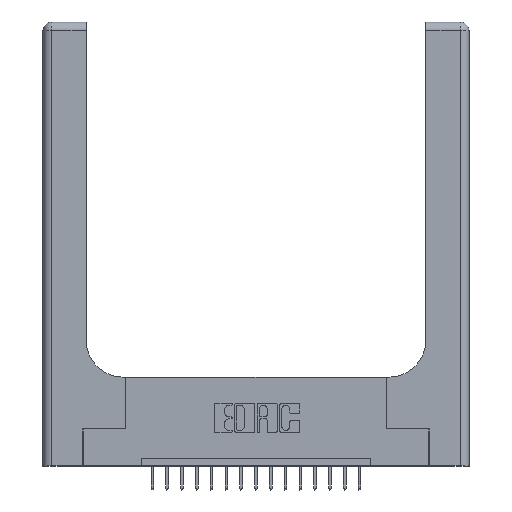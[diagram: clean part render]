
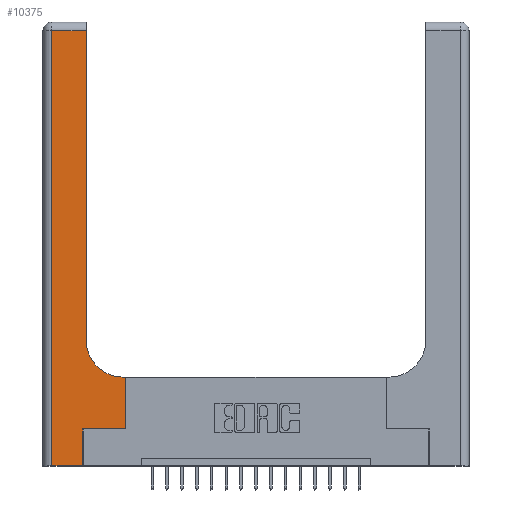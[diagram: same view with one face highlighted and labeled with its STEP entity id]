
A CAD part, top view. The second image highlights one B-rep face of the part: STEP entity #10375.
In plain terms, the highlighted planar face has unit normal (0, 0, 1).
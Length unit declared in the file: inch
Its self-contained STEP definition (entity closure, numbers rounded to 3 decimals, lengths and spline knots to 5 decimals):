
#289 = ORIENTED_EDGE ( 'NONE', *, *, #11114, .T. ) ;
#480 = DIRECTION ( 'NONE',  ( 1., 0., 0. ) ) ;
#503 = AXIS2_PLACEMENT_3D ( 'NONE', #3597, #14222, #6578 ) ;
#624 = LINE ( 'NONE', #5454, #6425 ) ;
#659 = DIRECTION ( 'NONE',  ( 1., 0., 0. ) ) ;
#871 = CARTESIAN_POINT ( 'NONE',  ( 0.269, 0., 0.37 ) ) ;
#910 = ORIENTED_EDGE ( 'NONE', *, *, #14593, .T. ) ;
#1097 = CIRCLE ( 'NONE', #3517, 0.25 ) ;
#1673 = EDGE_CURVE ( 'NONE', #16853, #19770, #10123, .T. ) ;
#1715 = DIRECTION ( 'NONE',  ( 0., 1., 0. ) ) ;
#1859 = EDGE_CURVE ( 'NONE', #10477, #11674, #624, .T. ) ;
#2254 = EDGE_CURVE ( 'NONE', #13086, #10477, #2289, .T. ) ;
#2289 = LINE ( 'NONE', #9511, #11050 ) ;
#2561 = EDGE_CURVE ( 'NONE', #14818, #2885, #15707, .T. ) ;
#2846 = ORIENTED_EDGE ( 'NONE', *, *, #12596, .T. ) ;
#2885 = VERTEX_POINT ( 'NONE', #14692 ) ;
#3455 = ORIENTED_EDGE ( 'NONE', *, *, #1859, .T. ) ;
#3517 = AXIS2_PLACEMENT_3D ( 'NONE', #14286, #15943, #480 ) ;
#3597 = CARTESIAN_POINT ( 'NONE',  ( 0., 3., 0.37 ) ) ;
#4347 = CARTESIAN_POINT ( 'NONE',  ( 0., 2.94, 0.37 ) ) ;
#4889 = LINE ( 'NONE', #10099, #17074 ) ;
#5375 = CARTESIAN_POINT ( 'NONE',  ( 0.5415, 0.6, 0.37 ) ) ;
#5384 = DIRECTION ( 'NONE',  ( 1., 0., 0. ) ) ;
#5454 = CARTESIAN_POINT ( 'NONE',  ( 0.269, 0.25, 0.37 ) ) ;
#5584 = LINE ( 'NONE', #13887, #9000 ) ;
#6143 = ORIENTED_EDGE ( 'NONE', *, *, #2561, .T. ) ;
#6267 = ORIENTED_EDGE ( 'NONE', *, *, #11590, .T. ) ;
#6387 = CARTESIAN_POINT ( 'NONE',  ( 0.06, 0., 0.37 ) ) ;
#6425 = VECTOR ( 'NONE', #5384, 39.37008 ) ;
#6578 = DIRECTION ( 'NONE',  ( -1., 0., 0. ) ) ;
#6607 = DIRECTION ( 'NONE',  ( 0., 1., 0. ) ) ;
#6799 = CARTESIAN_POINT ( 'NONE',  ( 0.5585, 0.25, 0.37 ) ) ;
#6810 = EDGE_CURVE ( 'NONE', #9966, #8165, #5584, .T. ) ;
#8165 = VERTEX_POINT ( 'NONE', #6387 ) ;
#8509 = VECTOR ( 'NONE', #6607, 39.37008 ) ;
#9000 = VECTOR ( 'NONE', #18345, 39.37008 ) ;
#9511 = CARTESIAN_POINT ( 'NONE',  ( 0.269, 0., 0.37 ) ) ;
#9547 = DIRECTION ( 'NONE',  ( -1., 0., 0. ) ) ;
#9689 = CARTESIAN_POINT ( 'NONE',  ( 0.2915, 0.6, 0.37 ) ) ;
#9756 = CARTESIAN_POINT ( 'NONE',  ( 0.2915, 0.85, 0.37 ) ) ;
#9778 = FACE_OUTER_BOUND ( 'NONE', #19981, .T. ) ;
#9915 = CARTESIAN_POINT ( 'NONE',  ( 0.269, 0.25, 0.37 ) ) ;
#9966 = VERTEX_POINT ( 'NONE', #16189 ) ;
#10099 = CARTESIAN_POINT ( 'NONE',  ( 0., 0., 0.37 ) ) ;
#10123 = LINE ( 'NONE', #9689, #14008 ) ;
#10139 = CARTESIAN_POINT ( 'NONE',  ( 0.2915, 3., 0.37 ) ) ;
#10203 = DIRECTION ( 'NONE',  ( 0., 1., 0. ) ) ;
#10375 = ADVANCED_FACE ( 'NONE', ( #9778 ), #15949, .F. ) ;
#10477 = VERTEX_POINT ( 'NONE', #9915 ) ;
#11050 = VECTOR ( 'NONE', #1715, 39.37008 ) ;
#11114 = EDGE_CURVE ( 'NONE', #8165, #13086, #4889, .T. ) ;
#11160 = LINE ( 'NONE', #4347, #18009 ) ;
#11544 = VECTOR ( 'NONE', #10203, 39.37008 ) ;
#11590 = EDGE_CURVE ( 'NONE', #11674, #16853, #18787, .T. ) ;
#11674 = VERTEX_POINT ( 'NONE', #11861 ) ;
#11861 = CARTESIAN_POINT ( 'NONE',  ( 0.5585, 0.25, 0.37 ) ) ;
#12596 = EDGE_CURVE ( 'NONE', #2885, #9966, #11160, .T. ) ;
#13086 = VERTEX_POINT ( 'NONE', #871 ) ;
#13156 = ORIENTED_EDGE ( 'NONE', *, *, #1673, .T. ) ;
#13887 = CARTESIAN_POINT ( 'NONE',  ( 0.06, 3., 0.37 ) ) ;
#14008 = VECTOR ( 'NONE', #9547, 39.37008 ) ;
#14222 = DIRECTION ( 'NONE',  ( 0., 0., -1. ) ) ;
#14286 = CARTESIAN_POINT ( 'NONE',  ( 0.5415, 0.85, 0.37 ) ) ;
#14593 = EDGE_CURVE ( 'NONE', #19770, #14818, #1097, .T. ) ;
#14692 = CARTESIAN_POINT ( 'NONE',  ( 0.2915, 2.94, 0.37 ) ) ;
#14818 = VERTEX_POINT ( 'NONE', #9756 ) ;
#15522 = DIRECTION ( 'NONE',  ( -1., 0., 0. ) ) ;
#15707 = LINE ( 'NONE', #10139, #11544 ) ;
#15943 = DIRECTION ( 'NONE',  ( 0., 0., -1. ) ) ;
#15949 = PLANE ( 'NONE',  #503 ) ;
#16189 = CARTESIAN_POINT ( 'NONE',  ( 0.06, 2.94, 0.37 ) ) ;
#16853 = VERTEX_POINT ( 'NONE', #19482 ) ;
#17074 = VECTOR ( 'NONE', #659, 39.37008 ) ;
#17922 = ORIENTED_EDGE ( 'NONE', *, *, #6810, .T. ) ;
#18009 = VECTOR ( 'NONE', #15522, 39.37008 ) ;
#18322 = ORIENTED_EDGE ( 'NONE', *, *, #2254, .T. ) ;
#18345 = DIRECTION ( 'NONE',  ( 0., -1., 0. ) ) ;
#18787 = LINE ( 'NONE', #6799, #8509 ) ;
#19482 = CARTESIAN_POINT ( 'NONE',  ( 0.5585, 0.6, 0.37 ) ) ;
#19770 = VERTEX_POINT ( 'NONE', #5375 ) ;
#19981 = EDGE_LOOP ( 'NONE', ( #6143, #2846, #17922, #289, #18322, #3455, #6267, #13156, #910 ) ) ;
